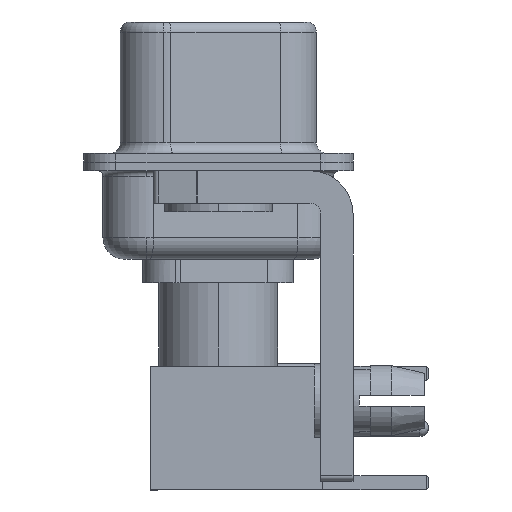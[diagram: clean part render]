
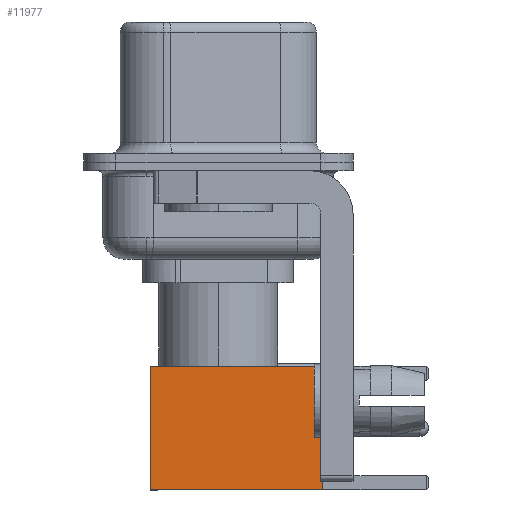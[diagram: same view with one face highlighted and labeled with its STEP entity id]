
A CAD part, left-side view. The second image highlights one B-rep face of the part: STEP entity #11977.
In plain terms, the highlighted face is planar.
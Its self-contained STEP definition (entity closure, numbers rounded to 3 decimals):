
#659 = VECTOR ( 'NONE', #21320, 1000. ) ;
#1380 = VERTEX_POINT ( 'NONE', #18087 ) ;
#1708 = EDGE_CURVE ( 'NONE', #5073, #1380, #26928, .T. ) ;
#1873 = VERTEX_POINT ( 'NONE', #19757 ) ;
#2571 = VERTEX_POINT ( 'NONE', #20788 ) ;
#2634 = VECTOR ( 'NONE', #12539, 1000. ) ;
#3594 = DIRECTION ( 'NONE',  ( -1., 0., 0. ) ) ;
#5073 = VERTEX_POINT ( 'NONE', #14389 ) ;
#10724 = LINE ( 'NONE', #12812, #2634 ) ;
#11977 = ADVANCED_FACE ( 'NONE', ( #20594 ), #14574, .T. ) ;
#12539 = DIRECTION ( 'NONE',  ( -1., 0., 0. ) ) ;
#12758 = EDGE_CURVE ( 'NONE', #2571, #1873, #10724, .T. ) ;
#12812 = CARTESIAN_POINT ( 'NONE',  ( 0., 2.875, 0. ) ) ;
#13416 = ORIENTED_EDGE ( 'NONE', *, *, #16939, .F. ) ;
#13798 = VECTOR ( 'NONE', #26762, 1000. ) ;
#14389 = CARTESIAN_POINT ( 'NONE',  ( 2.875, 2.875, 8. ) ) ;
#14574 = PLANE ( 'NONE',  #16865 ) ;
#15113 = ORIENTED_EDGE ( 'NONE', *, *, #12758, .T. ) ;
#16116 = DIRECTION ( 'NONE',  ( 0., 0., 1. ) ) ;
#16387 = CARTESIAN_POINT ( 'NONE',  ( 2.875, 2.875, 0. ) ) ;
#16634 = VECTOR ( 'NONE', #3594, 1000. ) ;
#16865 = AXIS2_PLACEMENT_3D ( 'NONE', #16387, #23104, #16116 ) ;
#16939 = EDGE_CURVE ( 'NONE', #1380, #1873, #22562, .T. ) ;
#17125 = CARTESIAN_POINT ( 'NONE',  ( 2.875, 2.875, 0. ) ) ;
#18087 = CARTESIAN_POINT ( 'NONE',  ( -2.875, 2.875, 8. ) ) ;
#19757 = CARTESIAN_POINT ( 'NONE',  ( -2.875, 2.875, 0. ) ) ;
#20311 = CARTESIAN_POINT ( 'NONE',  ( -2.875, 2.875, 0. ) ) ;
#20594 = FACE_OUTER_BOUND ( 'NONE', #24493, .T. ) ;
#20788 = CARTESIAN_POINT ( 'NONE',  ( 2.875, 2.875, 0. ) ) ;
#21320 = DIRECTION ( 'NONE',  ( 0., 0., -1. ) ) ;
#22427 = EDGE_CURVE ( 'NONE', #5073, #2571, #23710, .T. ) ;
#22562 = LINE ( 'NONE', #20311, #13798 ) ;
#23104 = DIRECTION ( 'NONE',  ( 0., 1., 0. ) ) ;
#23710 = LINE ( 'NONE', #17125, #659 ) ;
#24493 = EDGE_LOOP ( 'NONE', ( #27611, #15113, #13416, #26026 ) ) ;
#24691 = CARTESIAN_POINT ( 'NONE',  ( 0., 2.875, 8. ) ) ;
#26026 = ORIENTED_EDGE ( 'NONE', *, *, #1708, .F. ) ;
#26762 = DIRECTION ( 'NONE',  ( 0., 0., -1. ) ) ;
#26928 = LINE ( 'NONE', #24691, #16634 ) ;
#27611 = ORIENTED_EDGE ( 'NONE', *, *, #22427, .T. ) ;
